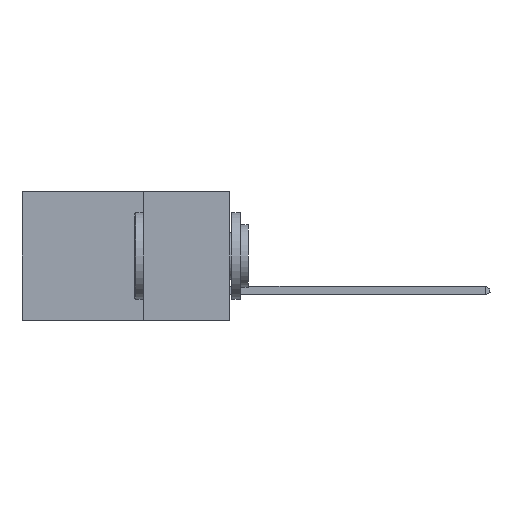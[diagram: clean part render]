
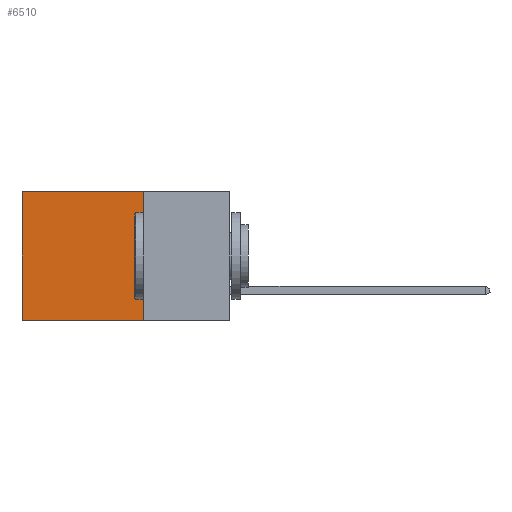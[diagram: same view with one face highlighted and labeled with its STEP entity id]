
A CAD part, left-side view. The second image highlights one B-rep face of the part: STEP entity #6510.
In plain terms, the highlighted planar face has unit normal (-1, 0, 0).
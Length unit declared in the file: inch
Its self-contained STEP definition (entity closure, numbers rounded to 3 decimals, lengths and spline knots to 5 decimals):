
#428 = CARTESIAN_POINT ( 'NONE',  ( 0.298, 0.6, 0. ) ) ;
#1414 = EDGE_CURVE ( 'NONE', #1480, #9607, #18770, .T. ) ;
#1480 = VERTEX_POINT ( 'NONE', #11666 ) ;
#1517 = VECTOR ( 'NONE', #3869, 39.37008 ) ;
#2061 = CARTESIAN_POINT ( 'NONE',  ( 0.298, 0.25, 0. ) ) ;
#3027 = PLANE ( 'NONE',  #7008 ) ;
#3097 = CARTESIAN_POINT ( 'NONE',  ( 0.298, 0.25, 0. ) ) ;
#3224 = VECTOR ( 'NONE', #7490, 39.37008 ) ;
#3869 = DIRECTION ( 'NONE',  ( 0., 1., 0. ) ) ;
#3951 = CARTESIAN_POINT ( 'NONE',  ( 0.298, 0.25, -0.37 ) ) ;
#4368 = EDGE_LOOP ( 'NONE', ( #14807, #5985, #13226, #9867 ) ) ;
#4497 = DIRECTION ( 'NONE',  ( 0., 1., 0. ) ) ;
#5185 = DIRECTION ( 'NONE',  ( 0., 0., -1. ) ) ;
#5556 = DIRECTION ( 'NONE',  ( 0., 0., -1. ) ) ;
#5985 = ORIENTED_EDGE ( 'NONE', *, *, #14063, .F. ) ;
#6070 = VECTOR ( 'NONE', #5556, 39.37008 ) ;
#6510 = ADVANCED_FACE ( 'NONE', ( #9418 ), #3027, .F. ) ;
#7008 = AXIS2_PLACEMENT_3D ( 'NONE', #3097, #13985, #5185 ) ;
#7176 = EDGE_CURVE ( 'NONE', #1480, #20364, #8013, .T. ) ;
#7225 = VERTEX_POINT ( 'NONE', #21452 ) ;
#7490 = DIRECTION ( 'NONE',  ( 0., 0., -1. ) ) ;
#8013 = LINE ( 'NONE', #2061, #6070 ) ;
#8511 = LINE ( 'NONE', #428, #3224 ) ;
#9416 = CARTESIAN_POINT ( 'NONE',  ( 0.298, 0.25, 0. ) ) ;
#9418 = FACE_OUTER_BOUND ( 'NONE', #4368, .T. ) ;
#9607 = VERTEX_POINT ( 'NONE', #11009 ) ;
#9867 = ORIENTED_EDGE ( 'NONE', *, *, #1414, .T. ) ;
#11009 = CARTESIAN_POINT ( 'NONE',  ( 0.298, 0.6, 0. ) ) ;
#11666 = CARTESIAN_POINT ( 'NONE',  ( 0.298, 0.25, 0. ) ) ;
#12272 = EDGE_CURVE ( 'NONE', #9607, #7225, #8511, .T. ) ;
#13226 = ORIENTED_EDGE ( 'NONE', *, *, #7176, .F. ) ;
#13985 = DIRECTION ( 'NONE',  ( 1., 0., 0. ) ) ;
#14063 = EDGE_CURVE ( 'NONE', #20364, #7225, #15705, .T. ) ;
#14282 = CARTESIAN_POINT ( 'NONE',  ( 0.298, 0.25, -0.37 ) ) ;
#14807 = ORIENTED_EDGE ( 'NONE', *, *, #12272, .T. ) ;
#15700 = VECTOR ( 'NONE', #4497, 39.37008 ) ;
#15705 = LINE ( 'NONE', #3951, #1517 ) ;
#18770 = LINE ( 'NONE', #9416, #15700 ) ;
#20364 = VERTEX_POINT ( 'NONE', #14282 ) ;
#21452 = CARTESIAN_POINT ( 'NONE',  ( 0.298, 0.6, -0.37 ) ) ;
